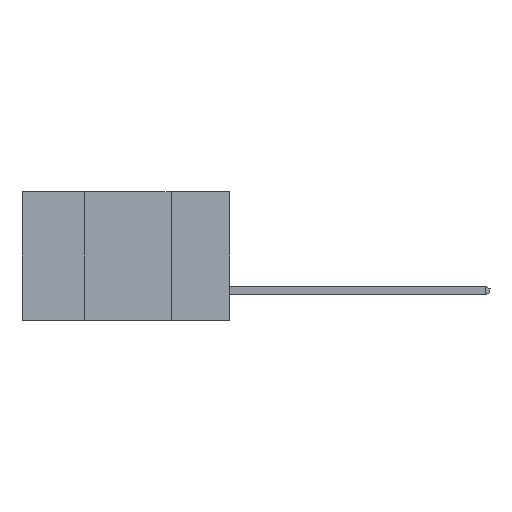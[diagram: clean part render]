
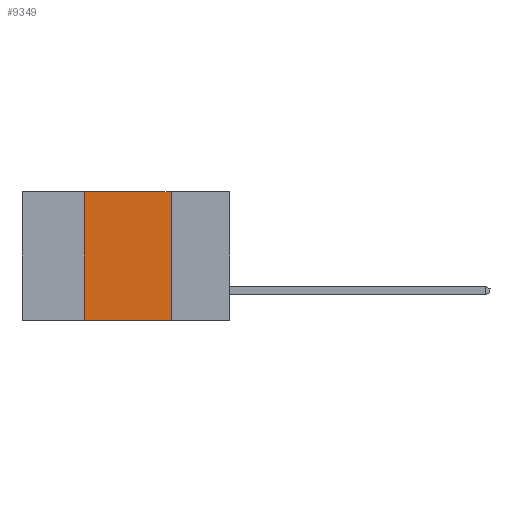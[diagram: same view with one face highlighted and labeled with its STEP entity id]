
A CAD part, left-side view. The second image highlights one B-rep face of the part: STEP entity #9349.
In plain terms, the highlighted planar face has unit normal (-1, 0, 0).
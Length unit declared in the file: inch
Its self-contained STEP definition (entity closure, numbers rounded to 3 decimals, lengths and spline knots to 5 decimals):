
#722 = CARTESIAN_POINT ( 'NONE',  ( 0., 0.6, 0. ) ) ;
#1031 = VECTOR ( 'NONE', #3096, 39.37008 ) ;
#1926 = CARTESIAN_POINT ( 'NONE',  ( 0., 0.42, -0.37 ) ) ;
#2058 = CARTESIAN_POINT ( 'NONE',  ( 0., 0.6, -0.37 ) ) ;
#2099 = DIRECTION ( 'NONE',  ( 0., -1., 0. ) ) ;
#2153 = CARTESIAN_POINT ( 'NONE',  ( 0., 0.42, 0. ) ) ;
#2168 = FACE_OUTER_BOUND ( 'NONE', #3053, .T. ) ;
#2242 = CARTESIAN_POINT ( 'NONE',  ( 0., 0.42, -0.37 ) ) ;
#2998 = EDGE_CURVE ( 'NONE', #9772, #6335, #8543, .T. ) ;
#3053 = EDGE_LOOP ( 'NONE', ( #4905, #5232, #3967, #5500 ) ) ;
#3096 = DIRECTION ( 'NONE',  ( 0., -1., 0. ) ) ;
#3302 = VERTEX_POINT ( 'NONE', #2242 ) ;
#3539 = LINE ( 'NONE', #1926, #7735 ) ;
#3967 = ORIENTED_EDGE ( 'NONE', *, *, #6184, .F. ) ;
#4159 = EDGE_CURVE ( 'NONE', #6335, #5546, #9072, .T. ) ;
#4629 = EDGE_CURVE ( 'NONE', #3302, #5546, #5303, .T. ) ;
#4905 = ORIENTED_EDGE ( 'NONE', *, *, #4159, .F. ) ;
#5232 = ORIENTED_EDGE ( 'NONE', *, *, #2998, .F. ) ;
#5303 = LINE ( 'NONE', #2058, #6622 ) ;
#5500 = ORIENTED_EDGE ( 'NONE', *, *, #4629, .T. ) ;
#5546 = VERTEX_POINT ( 'NONE', #6179 ) ;
#6179 = CARTESIAN_POINT ( 'NONE',  ( 0., 0.17, -0.37 ) ) ;
#6181 = DIRECTION ( 'NONE',  ( 1., 0., 0. ) ) ;
#6184 = EDGE_CURVE ( 'NONE', #3302, #9772, #3539, .T. ) ;
#6335 = VERTEX_POINT ( 'NONE', #6915 ) ;
#6622 = VECTOR ( 'NONE', #2099, 39.37008 ) ;
#6663 = DIRECTION ( 'NONE',  ( 0., 0., 1. ) ) ;
#6810 = CARTESIAN_POINT ( 'NONE',  ( 0., 0.6, 0. ) ) ;
#6855 = CARTESIAN_POINT ( 'NONE',  ( 0., 0.17, -0.37 ) ) ;
#6915 = CARTESIAN_POINT ( 'NONE',  ( 0., 0.17, 0. ) ) ;
#7521 = DIRECTION ( 'NONE',  ( 0., 0., -1. ) ) ;
#7731 = DIRECTION ( 'NONE',  ( 0., 0., -1. ) ) ;
#7735 = VECTOR ( 'NONE', #6663, 39.37008 ) ;
#8357 = PLANE ( 'NONE',  #10080 ) ;
#8543 = LINE ( 'NONE', #722, #1031 ) ;
#9072 = LINE ( 'NONE', #6855, #9412 ) ;
#9349 = ADVANCED_FACE ( 'NONE', ( #2168 ), #8357, .F. ) ;
#9412 = VECTOR ( 'NONE', #7521, 39.37008 ) ;
#9772 = VERTEX_POINT ( 'NONE', #2153 ) ;
#10080 = AXIS2_PLACEMENT_3D ( 'NONE', #6810, #6181, #7731 ) ;
